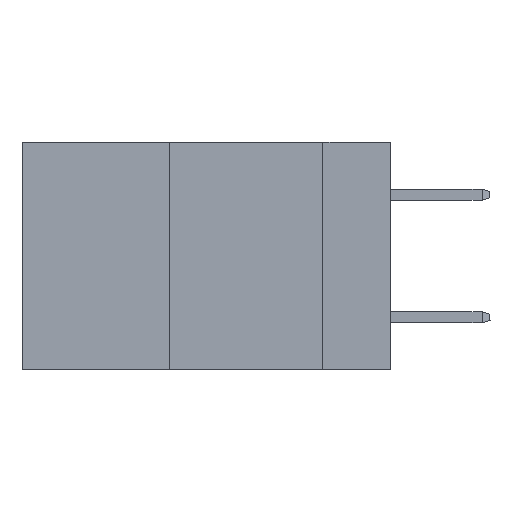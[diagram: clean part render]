
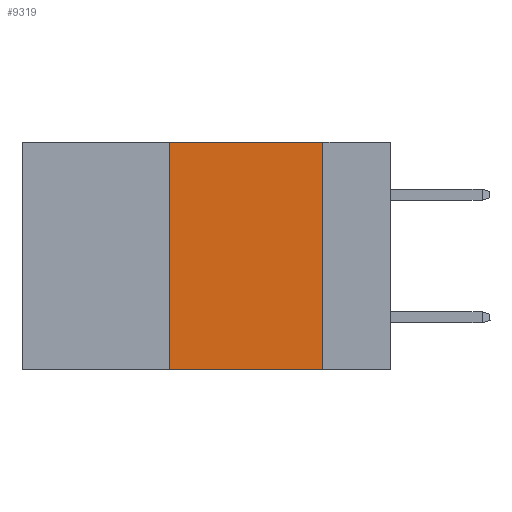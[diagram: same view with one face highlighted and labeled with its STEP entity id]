
A CAD part, left-side view. The second image highlights one B-rep face of the part: STEP entity #9319.
In plain terms, the highlighted planar face has unit normal (-1, 0, 0).
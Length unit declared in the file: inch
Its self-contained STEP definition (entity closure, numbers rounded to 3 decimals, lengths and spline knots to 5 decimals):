
#368 = CARTESIAN_POINT ( 'NONE',  ( 0., 0.36, 0. ) ) ;
#844 = CARTESIAN_POINT ( 'NONE',  ( 0., 0.11, -0.37 ) ) ;
#1584 = VERTEX_POINT ( 'NONE', #844 ) ;
#2871 = VECTOR ( 'NONE', #4694, 39.37008 ) ;
#4085 = PLANE ( 'NONE',  #5571 ) ;
#4569 = EDGE_CURVE ( 'NONE', #18992, #1584, #17316, .T. ) ;
#4694 = DIRECTION ( 'NONE',  ( 0., -1., 0. ) ) ;
#5053 = ORIENTED_EDGE ( 'NONE', *, *, #4569, .T. ) ;
#5571 = AXIS2_PLACEMENT_3D ( 'NONE', #8484, #14965, #19308 ) ;
#6825 = CARTESIAN_POINT ( 'NONE',  ( 0., 0.6, -0.37 ) ) ;
#7949 = EDGE_CURVE ( 'NONE', #18992, #10454, #16099, .T. ) ;
#8255 = FACE_OUTER_BOUND ( 'NONE', #22866, .T. ) ;
#8325 = ORIENTED_EDGE ( 'NONE', *, *, #7949, .F. ) ;
#8484 = CARTESIAN_POINT ( 'NONE',  ( 0., 0.6, 0. ) ) ;
#9257 = VERTEX_POINT ( 'NONE', #24405 ) ;
#9319 = ADVANCED_FACE ( 'NONE', ( #8255 ), #4085, .F. ) ;
#10454 = VERTEX_POINT ( 'NONE', #368 ) ;
#11167 = EDGE_CURVE ( 'NONE', #9257, #1584, #14512, .T. ) ;
#13138 = CARTESIAN_POINT ( 'NONE',  ( 0., 0.6, 0. ) ) ;
#13632 = VECTOR ( 'NONE', #26554, 39.37008 ) ;
#14383 = VECTOR ( 'NONE', #22676, 39.37008 ) ;
#14512 = LINE ( 'NONE', #14717, #17551 ) ;
#14552 = ORIENTED_EDGE ( 'NONE', *, *, #11167, .F. ) ;
#14717 = CARTESIAN_POINT ( 'NONE',  ( 0., 0.11, 0. ) ) ;
#14965 = DIRECTION ( 'NONE',  ( 1., 0., 0. ) ) ;
#16099 = LINE ( 'NONE', #16643, #14383 ) ;
#16643 = CARTESIAN_POINT ( 'NONE',  ( 0., 0.36, 0. ) ) ;
#17316 = LINE ( 'NONE', #6825, #2871 ) ;
#17551 = VECTOR ( 'NONE', #19146, 39.37008 ) ;
#17607 = ORIENTED_EDGE ( 'NONE', *, *, #17896, .F. ) ;
#17896 = EDGE_CURVE ( 'NONE', #10454, #9257, #20392, .T. ) ;
#18992 = VERTEX_POINT ( 'NONE', #21842 ) ;
#19146 = DIRECTION ( 'NONE',  ( 0., 0., -1. ) ) ;
#19308 = DIRECTION ( 'NONE',  ( 0., 0., -1. ) ) ;
#20392 = LINE ( 'NONE', #13138, #13632 ) ;
#21842 = CARTESIAN_POINT ( 'NONE',  ( 0., 0.36, -0.37 ) ) ;
#22676 = DIRECTION ( 'NONE',  ( 0., 0., 1. ) ) ;
#22866 = EDGE_LOOP ( 'NONE', ( #14552, #17607, #8325, #5053 ) ) ;
#24405 = CARTESIAN_POINT ( 'NONE',  ( 0., 0.11, 0. ) ) ;
#26554 = DIRECTION ( 'NONE',  ( 0., -1., 0. ) ) ;
